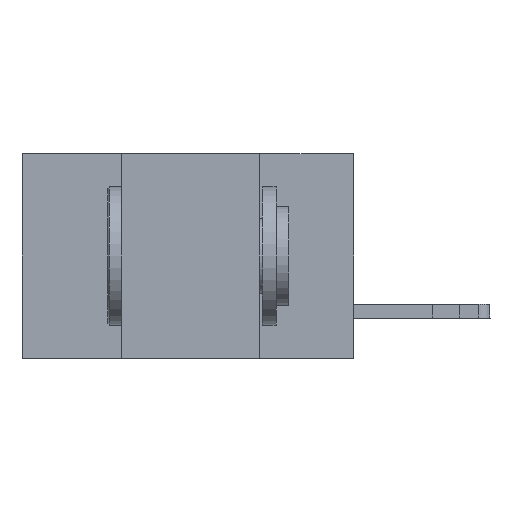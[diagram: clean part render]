
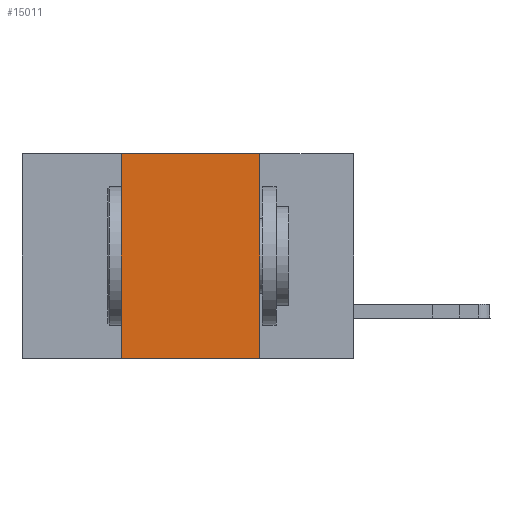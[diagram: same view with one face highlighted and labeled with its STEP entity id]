
A CAD part, left-side view. The second image highlights one B-rep face of the part: STEP entity #15011.
In plain terms, the highlighted planar face has unit normal (-1, 0, 0).
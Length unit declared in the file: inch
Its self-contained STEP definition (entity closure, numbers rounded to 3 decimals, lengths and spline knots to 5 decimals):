
#852 = PLANE ( 'NONE',  #6498 ) ;
#1172 = EDGE_CURVE ( 'NONE', #13685, #1305, #19580, .T. ) ;
#1305 = VERTEX_POINT ( 'NONE', #12607 ) ;
#1669 = ORIENTED_EDGE ( 'NONE', *, *, #14815, .F. ) ;
#1962 = ORIENTED_EDGE ( 'NONE', *, *, #12140, .F. ) ;
#2001 = LINE ( 'NONE', #16283, #3815 ) ;
#2513 = DIRECTION ( 'NONE',  ( 1., 0., 0. ) ) ;
#2730 = ORIENTED_EDGE ( 'NONE', *, *, #1172, .F. ) ;
#3815 = VECTOR ( 'NONE', #6792, 39.37008 ) ;
#4177 = FACE_OUTER_BOUND ( 'NONE', #6192, .T. ) ;
#4753 = VECTOR ( 'NONE', #13627, 39.37008 ) ;
#5300 = CARTESIAN_POINT ( 'NONE',  ( 0., 0.17, 0. ) ) ;
#5959 = VERTEX_POINT ( 'NONE', #18471 ) ;
#6101 = CARTESIAN_POINT ( 'NONE',  ( 0., 0.17, 0. ) ) ;
#6192 = EDGE_LOOP ( 'NONE', ( #2730, #1962, #1669, #18104 ) ) ;
#6498 = AXIS2_PLACEMENT_3D ( 'NONE', #7214, #2513, #15441 ) ;
#6792 = DIRECTION ( 'NONE',  ( 0., 0., 1. ) ) ;
#7214 = CARTESIAN_POINT ( 'NONE',  ( 0., 0.6, 0. ) ) ;
#7462 = CARTESIAN_POINT ( 'NONE',  ( 0., 0.6, -0.37 ) ) ;
#7648 = VECTOR ( 'NONE', #13548, 39.37008 ) ;
#9208 = VECTOR ( 'NONE', #16626, 39.37008 ) ;
#10279 = LINE ( 'NONE', #11724, #9208 ) ;
#11724 = CARTESIAN_POINT ( 'NONE',  ( 0., 0.6, 0. ) ) ;
#12140 = EDGE_CURVE ( 'NONE', #15963, #13685, #10279, .T. ) ;
#12607 = CARTESIAN_POINT ( 'NONE',  ( 0., 0.17, -0.37 ) ) ;
#12699 = CARTESIAN_POINT ( 'NONE',  ( 0., 0.42, 0. ) ) ;
#13548 = DIRECTION ( 'NONE',  ( 0., 0., -1. ) ) ;
#13627 = DIRECTION ( 'NONE',  ( 0., -1., 0. ) ) ;
#13671 = EDGE_CURVE ( 'NONE', #5959, #1305, #20375, .T. ) ;
#13685 = VERTEX_POINT ( 'NONE', #6101 ) ;
#14815 = EDGE_CURVE ( 'NONE', #5959, #15963, #2001, .T. ) ;
#15011 = ADVANCED_FACE ( 'NONE', ( #4177 ), #852, .F. ) ;
#15441 = DIRECTION ( 'NONE',  ( 0., 0., -1. ) ) ;
#15963 = VERTEX_POINT ( 'NONE', #12699 ) ;
#16283 = CARTESIAN_POINT ( 'NONE',  ( 0., 0.42, 0. ) ) ;
#16626 = DIRECTION ( 'NONE',  ( 0., -1., 0. ) ) ;
#18104 = ORIENTED_EDGE ( 'NONE', *, *, #13671, .T. ) ;
#18471 = CARTESIAN_POINT ( 'NONE',  ( 0., 0.42, -0.37 ) ) ;
#19580 = LINE ( 'NONE', #5300, #7648 ) ;
#20375 = LINE ( 'NONE', #7462, #4753 ) ;
